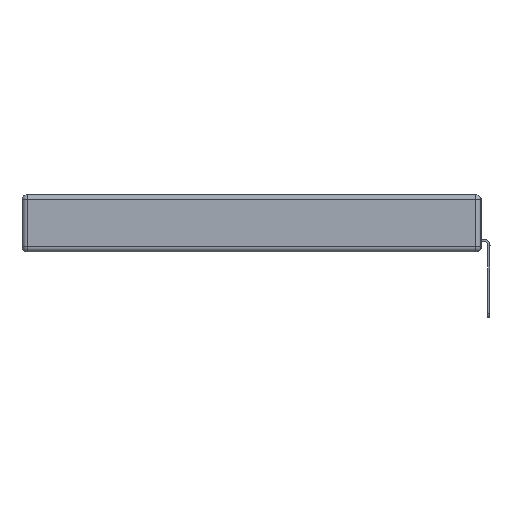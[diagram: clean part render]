
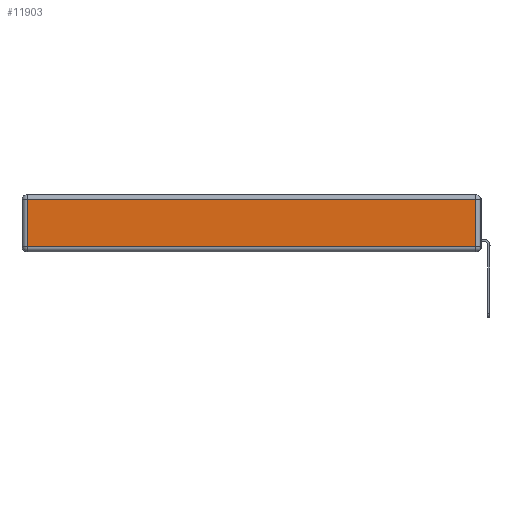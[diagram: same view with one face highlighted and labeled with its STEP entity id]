
A CAD part, left-side view. The second image highlights one B-rep face of the part: STEP entity #11903.
In plain terms, the highlighted planar face has unit normal (-1, 0, 0).
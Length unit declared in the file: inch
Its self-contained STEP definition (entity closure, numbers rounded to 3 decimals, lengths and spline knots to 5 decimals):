
#203 = VERTEX_POINT ( 'NONE', #12150 ) ;
#660 = CARTESIAN_POINT ( 'NONE',  ( 0., 2.72, -0.313 ) ) ;
#718 = CARTESIAN_POINT ( 'NONE',  ( 0., 2.75, -0.03 ) ) ;
#850 = VECTOR ( 'NONE', #1883, 39.37008 ) ;
#954 = LINE ( 'NONE', #5618, #11469 ) ;
#1148 = VERTEX_POINT ( 'NONE', #660 ) ;
#1171 = ORIENTED_EDGE ( 'NONE', *, *, #10264, .T. ) ;
#1883 = DIRECTION ( 'NONE',  ( 0., 1., 0. ) ) ;
#2092 = FACE_OUTER_BOUND ( 'NONE', #10125, .T. ) ;
#2629 = LINE ( 'NONE', #718, #850 ) ;
#2784 = CARTESIAN_POINT ( 'NONE',  ( 0., 0.03, -0.313 ) ) ;
#2834 = EDGE_CURVE ( 'NONE', #8286, #1148, #4295, .T. ) ;
#3854 = DIRECTION ( 'NONE',  ( 0., 0., 1. ) ) ;
#3981 = VECTOR ( 'NONE', #6756, 39.37008 ) ;
#4295 = LINE ( 'NONE', #12807, #3981 ) ;
#5362 = DIRECTION ( 'NONE',  ( 0., 0., 1. ) ) ;
#5618 = CARTESIAN_POINT ( 'NONE',  ( 0., 0., -0.313 ) ) ;
#5779 = LINE ( 'NONE', #12472, #10873 ) ;
#5894 = EDGE_CURVE ( 'NONE', #8923, #203, #5779, .T. ) ;
#6756 = DIRECTION ( 'NONE',  ( 0., 0., -1. ) ) ;
#7780 = DIRECTION ( 'NONE',  ( -1., 0., 0. ) ) ;
#8286 = VERTEX_POINT ( 'NONE', #12090 ) ;
#8524 = DIRECTION ( 'NONE',  ( 0., -1., 0. ) ) ;
#8769 = ORIENTED_EDGE ( 'NONE', *, *, #5894, .T. ) ;
#8923 = VERTEX_POINT ( 'NONE', #2784 ) ;
#9001 = CARTESIAN_POINT ( 'NONE',  ( 0., 0., -0.343 ) ) ;
#10125 = EDGE_LOOP ( 'NONE', ( #12509, #8769, #1171, #11133 ) ) ;
#10264 = EDGE_CURVE ( 'NONE', #203, #8286, #2629, .T. ) ;
#10847 = PLANE ( 'NONE',  #10915 ) ;
#10873 = VECTOR ( 'NONE', #5362, 39.37008 ) ;
#10915 = AXIS2_PLACEMENT_3D ( 'NONE', #9001, #7780, #3854 ) ;
#11133 = ORIENTED_EDGE ( 'NONE', *, *, #2834, .T. ) ;
#11469 = VECTOR ( 'NONE', #8524, 39.37008 ) ;
#11903 = ADVANCED_FACE ( 'NONE', ( #2092 ), #10847, .T. ) ;
#12090 = CARTESIAN_POINT ( 'NONE',  ( 0., 2.72, -0.03 ) ) ;
#12150 = CARTESIAN_POINT ( 'NONE',  ( 0., 0.03, -0.03 ) ) ;
#12472 = CARTESIAN_POINT ( 'NONE',  ( 0., 0.03, -0.343 ) ) ;
#12509 = ORIENTED_EDGE ( 'NONE', *, *, #12632, .T. ) ;
#12632 = EDGE_CURVE ( 'NONE', #1148, #8923, #954, .T. ) ;
#12807 = CARTESIAN_POINT ( 'NONE',  ( 0., 2.72, -0.343 ) ) ;
